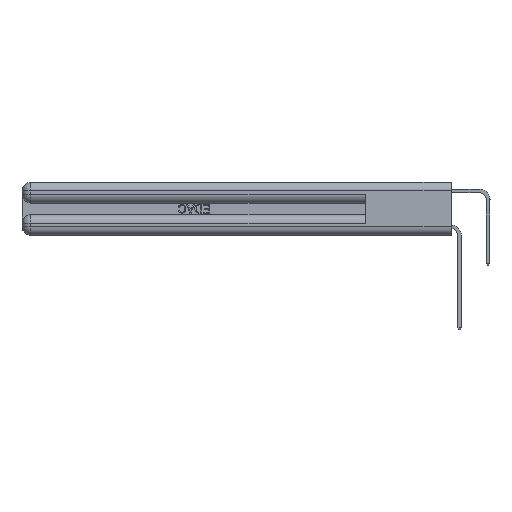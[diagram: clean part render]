
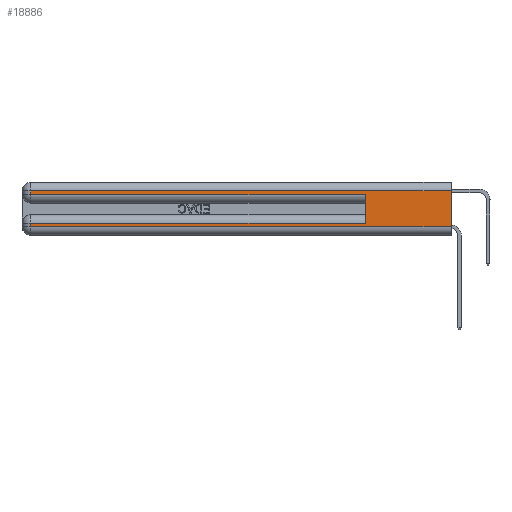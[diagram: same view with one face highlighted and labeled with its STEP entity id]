
A CAD part, left-side view. The second image highlights one B-rep face of the part: STEP entity #18886.
In plain terms, the highlighted planar face has unit normal (-1, 0, 0).
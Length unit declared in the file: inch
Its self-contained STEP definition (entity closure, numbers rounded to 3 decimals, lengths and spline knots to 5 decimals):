
#137 = AXIS2_PLACEMENT_3D ( 'NONE', #19507, #16233, #33413 ) ;
#939 = LINE ( 'NONE', #33906, #6744 ) ;
#1763 = DIRECTION ( 'NONE',  ( 0., 0., 1. ) ) ;
#2115 = VERTEX_POINT ( 'NONE', #30914 ) ;
#2214 = CARTESIAN_POINT ( 'NONE',  ( 0., 0., 0.31 ) ) ;
#3806 = EDGE_CURVE ( 'NONE', #17519, #4761, #21427, .T. ) ;
#4307 = ORIENTED_EDGE ( 'NONE', *, *, #25589, .F. ) ;
#4761 = VERTEX_POINT ( 'NONE', #35966 ) ;
#4870 = ORIENTED_EDGE ( 'NONE', *, *, #35796, .F. ) ;
#6744 = VECTOR ( 'NONE', #20719, 39.37008 ) ;
#7209 = VERTEX_POINT ( 'NONE', #9197 ) ;
#7659 = CARTESIAN_POINT ( 'NONE',  ( 0., 0., 0.285 ) ) ;
#9132 = VERTEX_POINT ( 'NONE', #12484 ) ;
#9197 = CARTESIAN_POINT ( 'NONE',  ( 0., 0., 0.06 ) ) ;
#10353 = CARTESIAN_POINT ( 'NONE',  ( 0., 2.94, 0.31 ) ) ;
#10467 = DIRECTION ( 'NONE',  ( 0., 0., -1. ) ) ;
#10892 = VERTEX_POINT ( 'NONE', #11675 ) ;
#11675 = CARTESIAN_POINT ( 'NONE',  ( 0., 2.94, 0.06 ) ) ;
#12387 = ORIENTED_EDGE ( 'NONE', *, *, #27353, .T. ) ;
#12484 = CARTESIAN_POINT ( 'NONE',  ( 0., 0.6, 0.085 ) ) ;
#15406 = DIRECTION ( 'NONE',  ( 0., 0., -1. ) ) ;
#16233 = DIRECTION ( 'NONE',  ( 1., 0., 0. ) ) ;
#16363 = PLANE ( 'NONE',  #137 ) ;
#16633 = LINE ( 'NONE', #2214, #36797 ) ;
#17519 = VERTEX_POINT ( 'NONE', #30171 ) ;
#17860 = EDGE_CURVE ( 'NONE', #10892, #7209, #939, .T. ) ;
#18750 = CARTESIAN_POINT ( 'NONE',  ( 0., 0.6, 0.145 ) ) ;
#18886 = ADVANCED_FACE ( 'NONE', ( #22315 ), #16363, .F. ) ;
#19097 = DIRECTION ( 'NONE',  ( 0., 1., 0. ) ) ;
#19252 = CARTESIAN_POINT ( 'NONE',  ( 0., 0., 0.085 ) ) ;
#19507 = CARTESIAN_POINT ( 'NONE',  ( 0., 0., 0.37 ) ) ;
#20719 = DIRECTION ( 'NONE',  ( 0., -1., 0. ) ) ;
#20821 = VECTOR ( 'NONE', #1763, 39.37008 ) ;
#21215 = VERTEX_POINT ( 'NONE', #30030 ) ;
#21427 = LINE ( 'NONE', #7659, #24108 ) ;
#21814 = VECTOR ( 'NONE', #10467, 39.37008 ) ;
#21993 = DIRECTION ( 'NONE',  ( 0., 0., -1. ) ) ;
#22315 = FACE_OUTER_BOUND ( 'NONE', #32992, .T. ) ;
#22857 = EDGE_CURVE ( 'NONE', #9132, #2115, #27424, .T. ) ;
#23323 = EDGE_CURVE ( 'NONE', #21215, #24591, #16633, .T. ) ;
#24108 = VECTOR ( 'NONE', #30547, 39.37008 ) ;
#24291 = ORIENTED_EDGE ( 'NONE', *, *, #17860, .T. ) ;
#24489 = VECTOR ( 'NONE', #21993, 39.37008 ) ;
#24591 = VERTEX_POINT ( 'NONE', #10353 ) ;
#24682 = EDGE_CURVE ( 'NONE', #24591, #17519, #31629, .T. ) ;
#25085 = CARTESIAN_POINT ( 'NONE',  ( 0., 2.94, 0.37 ) ) ;
#25400 = DIRECTION ( 'NONE',  ( 0., 1., 0. ) ) ;
#25589 = EDGE_CURVE ( 'NONE', #9132, #4761, #36505, .T. ) ;
#27353 = EDGE_CURVE ( 'NONE', #2115, #10892, #27854, .T. ) ;
#27424 = LINE ( 'NONE', #19252, #34569 ) ;
#27672 = ORIENTED_EDGE ( 'NONE', *, *, #24682, .T. ) ;
#27854 = LINE ( 'NONE', #32706, #30972 ) ;
#28552 = ORIENTED_EDGE ( 'NONE', *, *, #22857, .T. ) ;
#29124 = ORIENTED_EDGE ( 'NONE', *, *, #23323, .T. ) ;
#29529 = ORIENTED_EDGE ( 'NONE', *, *, #3806, .T. ) ;
#30030 = CARTESIAN_POINT ( 'NONE',  ( 0., 0., 0.31 ) ) ;
#30171 = CARTESIAN_POINT ( 'NONE',  ( 0., 2.94, 0.285 ) ) ;
#30547 = DIRECTION ( 'NONE',  ( 0., -1., 0. ) ) ;
#30727 = CARTESIAN_POINT ( 'NONE',  ( 0., 0., 0.37 ) ) ;
#30914 = CARTESIAN_POINT ( 'NONE',  ( 0., 2.94, 0.085 ) ) ;
#30972 = VECTOR ( 'NONE', #15406, 39.37008 ) ;
#31629 = LINE ( 'NONE', #25085, #21814 ) ;
#32103 = LINE ( 'NONE', #30727, #24489 ) ;
#32706 = CARTESIAN_POINT ( 'NONE',  ( 0., 2.94, 0.37 ) ) ;
#32992 = EDGE_LOOP ( 'NONE', ( #4870, #29124, #27672, #29529, #4307, #28552, #12387, #24291 ) ) ;
#33413 = DIRECTION ( 'NONE',  ( 0., 0., -1. ) ) ;
#33906 = CARTESIAN_POINT ( 'NONE',  ( 0., 0., 0.06 ) ) ;
#34569 = VECTOR ( 'NONE', #25400, 39.37008 ) ;
#35796 = EDGE_CURVE ( 'NONE', #21215, #7209, #32103, .T. ) ;
#35966 = CARTESIAN_POINT ( 'NONE',  ( 0., 0.6, 0.285 ) ) ;
#36505 = LINE ( 'NONE', #18750, #20821 ) ;
#36797 = VECTOR ( 'NONE', #19097, 39.37008 ) ;
